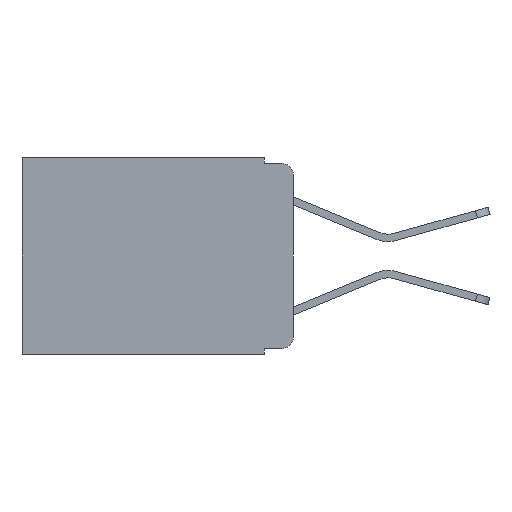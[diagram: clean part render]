
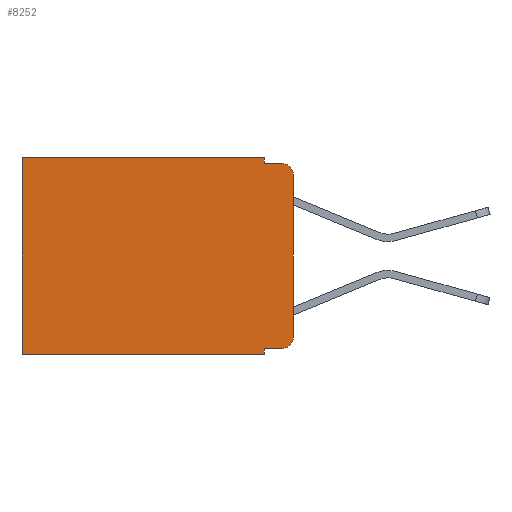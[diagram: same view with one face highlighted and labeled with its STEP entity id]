
A CAD part, left-side view. The second image highlights one B-rep face of the part: STEP entity #8252.
In plain terms, the highlighted planar face has unit normal (-1, 0, 0).
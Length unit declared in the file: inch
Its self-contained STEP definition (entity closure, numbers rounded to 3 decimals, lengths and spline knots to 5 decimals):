
#71 = ORIENTED_EDGE ( 'NONE', *, *, #12678, .T. ) ;
#135 = CARTESIAN_POINT ( 'NONE',  ( 0.298, 0.02, -0.313 ) ) ;
#393 = VERTEX_POINT ( 'NONE', #16070 ) ;
#530 = VERTEX_POINT ( 'NONE', #12077 ) ;
#570 = EDGE_CURVE ( 'NONE', #14832, #3366, #2779, .T. ) ;
#741 = DIRECTION ( 'NONE',  ( 0., 1., 0. ) ) ;
#866 = CARTESIAN_POINT ( 'NONE',  ( 0.298, 0.051, 0. ) ) ;
#1326 = CARTESIAN_POINT ( 'NONE',  ( 0.298, 0., -0.343 ) ) ;
#1462 = CARTESIAN_POINT ( 'NONE',  ( 0.298, 0.473, -0.343 ) ) ;
#1668 = PLANE ( 'NONE',  #9747 ) ;
#1699 = ORIENTED_EDGE ( 'NONE', *, *, #5178, .T. ) ;
#1999 = ORIENTED_EDGE ( 'NONE', *, *, #570, .T. ) ;
#2048 = VECTOR ( 'NONE', #20413, 39.37008 ) ;
#2599 = VECTOR ( 'NONE', #20903, 39.37008 ) ;
#2779 = CIRCLE ( 'NONE', #21078, 0.02 ) ;
#3121 = CARTESIAN_POINT ( 'NONE',  ( 0.298, 0., -0.313 ) ) ;
#3366 = VERTEX_POINT ( 'NONE', #3121 ) ;
#3381 = DIRECTION ( 'NONE',  ( 0., 0., -1. ) ) ;
#3601 = VERTEX_POINT ( 'NONE', #12918 ) ;
#3815 = DIRECTION ( 'NONE',  ( 0., -1., 0. ) ) ;
#3845 = ORIENTED_EDGE ( 'NONE', *, *, #19138, .F. ) ;
#4125 = ORIENTED_EDGE ( 'NONE', *, *, #9703, .F. ) ;
#4245 = EDGE_CURVE ( 'NONE', #19791, #17239, #16791, .T. ) ;
#4258 = DIRECTION ( 'NONE',  ( -1., 0., 0. ) ) ;
#4418 = EDGE_LOOP ( 'NONE', ( #4125, #71, #16992, #11523, #14790, #13061, #11789, #3845, #1699, #1999 ) ) ;
#5178 = EDGE_CURVE ( 'NONE', #393, #14832, #20446, .T. ) ;
#6208 = DIRECTION ( 'NONE',  ( 0., -1., 0. ) ) ;
#6727 = LINE ( 'NONE', #15475, #15796 ) ;
#7011 = LINE ( 'NONE', #866, #2048 ) ;
#7975 = CARTESIAN_POINT ( 'NONE',  ( 0.298, 0.051, -0.333 ) ) ;
#7978 = CARTESIAN_POINT ( 'NONE',  ( 0.298, 0.051, -0.01 ) ) ;
#8252 = ADVANCED_FACE ( 'NONE', ( #11427 ), #1668, .F. ) ;
#8851 = DIRECTION ( 'NONE',  ( -1., 0., 0. ) ) ;
#9703 = EDGE_CURVE ( 'NONE', #20722, #3366, #11368, .T. ) ;
#9747 = AXIS2_PLACEMENT_3D ( 'NONE', #19488, #13175, #3381 ) ;
#9820 = AXIS2_PLACEMENT_3D ( 'NONE', #18415, #8851, #20007 ) ;
#10149 = EDGE_CURVE ( 'NONE', #530, #19791, #7011, .T. ) ;
#10300 = CARTESIAN_POINT ( 'NONE',  ( 0.298, 0.051, -0.01 ) ) ;
#11368 = LINE ( 'NONE', #17827, #2599 ) ;
#11427 = FACE_OUTER_BOUND ( 'NONE', #4418, .T. ) ;
#11523 = ORIENTED_EDGE ( 'NONE', *, *, #10149, .F. ) ;
#11789 = ORIENTED_EDGE ( 'NONE', *, *, #17961, .F. ) ;
#11808 = LINE ( 'NONE', #12484, #14033 ) ;
#12077 = CARTESIAN_POINT ( 'NONE',  ( 0.298, 0.051, 0. ) ) ;
#12222 = VECTOR ( 'NONE', #13934, 39.37008 ) ;
#12349 = CARTESIAN_POINT ( 'NONE',  ( 0.298, 0.473, 0. ) ) ;
#12484 = CARTESIAN_POINT ( 'NONE',  ( 0.298, 0.051, 0. ) ) ;
#12568 = VECTOR ( 'NONE', #3815, 39.37008 ) ;
#12678 = EDGE_CURVE ( 'NONE', #20722, #17239, #20190, .T. ) ;
#12879 = DIRECTION ( 'NONE',  ( 0., 1., 0. ) ) ;
#12918 = CARTESIAN_POINT ( 'NONE',  ( 0.298, 0.051, -0.343 ) ) ;
#13061 = ORIENTED_EDGE ( 'NONE', *, *, #13947, .T. ) ;
#13175 = DIRECTION ( 'NONE',  ( 1., 0., 0. ) ) ;
#13205 = LINE ( 'NONE', #12349, #12222 ) ;
#13934 = DIRECTION ( 'NONE',  ( 0., 0., -1. ) ) ;
#13947 = EDGE_CURVE ( 'NONE', #19589, #17471, #13205, .T. ) ;
#14033 = VECTOR ( 'NONE', #14080, 39.37008 ) ;
#14080 = DIRECTION ( 'NONE',  ( 0., 0., -1. ) ) ;
#14534 = CARTESIAN_POINT ( 'NONE',  ( 0.298, 0.02, -0.333 ) ) ;
#14790 = ORIENTED_EDGE ( 'NONE', *, *, #17845, .T. ) ;
#14832 = VERTEX_POINT ( 'NONE', #14534 ) ;
#15475 = CARTESIAN_POINT ( 'NONE',  ( 0.298, 0., 0. ) ) ;
#15796 = VECTOR ( 'NONE', #741, 39.37008 ) ;
#16070 = CARTESIAN_POINT ( 'NONE',  ( 0.298, 0.051, -0.333 ) ) ;
#16536 = VECTOR ( 'NONE', #12879, 39.37008 ) ;
#16589 = DIRECTION ( 'NONE',  ( 0., 0., -1. ) ) ;
#16791 = LINE ( 'NONE', #10300, #12568 ) ;
#16992 = ORIENTED_EDGE ( 'NONE', *, *, #4245, .F. ) ;
#17239 = VERTEX_POINT ( 'NONE', #18683 ) ;
#17471 = VERTEX_POINT ( 'NONE', #1462 ) ;
#17827 = CARTESIAN_POINT ( 'NONE',  ( 0.298, 0., 0. ) ) ;
#17845 = EDGE_CURVE ( 'NONE', #530, #19589, #6727, .T. ) ;
#17961 = EDGE_CURVE ( 'NONE', #3601, #17471, #20715, .T. ) ;
#18415 = CARTESIAN_POINT ( 'NONE',  ( 0.298, 0.02, -0.03 ) ) ;
#18635 = CARTESIAN_POINT ( 'NONE',  ( 0.298, 0.473, 0. ) ) ;
#18683 = CARTESIAN_POINT ( 'NONE',  ( 0.298, 0.02, -0.01 ) ) ;
#19138 = EDGE_CURVE ( 'NONE', #393, #3601, #11808, .T. ) ;
#19488 = CARTESIAN_POINT ( 'NONE',  ( 0.298, 0., 0. ) ) ;
#19589 = VERTEX_POINT ( 'NONE', #18635 ) ;
#19791 = VERTEX_POINT ( 'NONE', #7978 ) ;
#19901 = CARTESIAN_POINT ( 'NONE',  ( 0.298, 0., -0.03 ) ) ;
#20007 = DIRECTION ( 'NONE',  ( 0., 0., -1. ) ) ;
#20190 = CIRCLE ( 'NONE', #9820, 0.02 ) ;
#20413 = DIRECTION ( 'NONE',  ( 0., 0., -1. ) ) ;
#20446 = LINE ( 'NONE', #7975, #20925 ) ;
#20715 = LINE ( 'NONE', #1326, #16536 ) ;
#20722 = VERTEX_POINT ( 'NONE', #19901 ) ;
#20903 = DIRECTION ( 'NONE',  ( 0., 0., -1. ) ) ;
#20925 = VECTOR ( 'NONE', #6208, 39.37008 ) ;
#21078 = AXIS2_PLACEMENT_3D ( 'NONE', #135, #4258, #16589 ) ;
